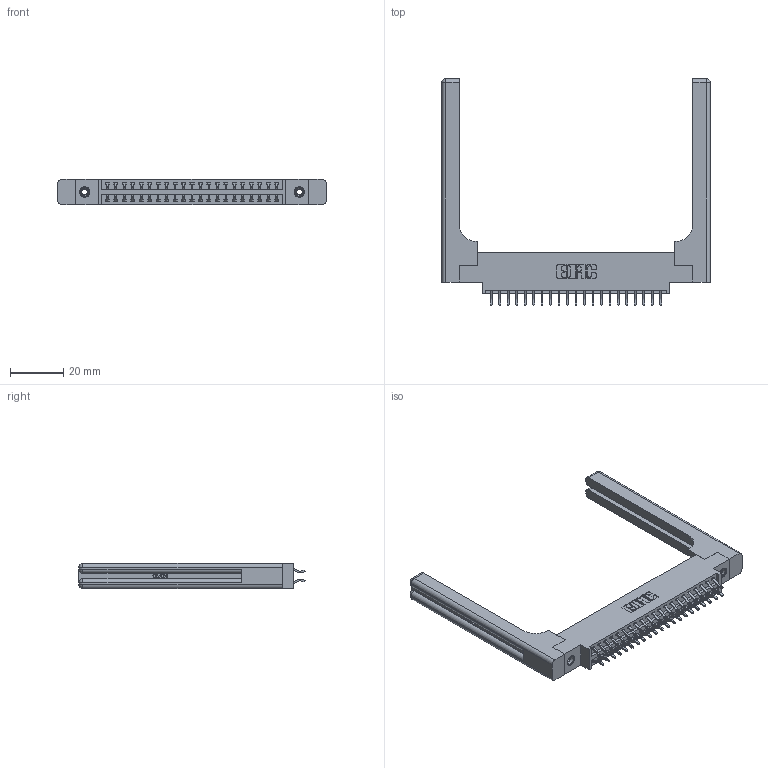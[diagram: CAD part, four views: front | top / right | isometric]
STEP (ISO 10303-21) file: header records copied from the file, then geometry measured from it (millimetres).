
FILE_DESCRIPTION (( 'STEP AP203' ), '1' );
FILE_NAME ('346-042-556-858.STEP', '2022-05-20T05:15:51', ( '' ), ( '' ), 'SwSTEP 2.0', 'SolidWorks 2020', '' );
FILE_SCHEMA (( 'CONFIG_CONTROL_DESIGN' ));
Length unit declared in the file: inch
Products named in the file (5): 346-220-058_345-220-058; 345-292-001_556 Tail; 345-250-001_345-250-001-102; 346-042-556-858; 346 Part_0.170 Offset - 0.156 Dia-TH
Assembly tree (47 placements, depth 2):
  346-042-556-858
    346 Part_0.170 Offset - 0.156 Dia-TH
    345-292-001_556 Tail  x42
    345-250-001_345-250-001-102  x2
    346-220-058_345-220-058  x2
Bounding box: 100.74 x 84.84 x 9.4 mm (x, y, z)
Volume: 16979.8 mm3; surface area: 17856.4 mm2
Topology: 47 solids, 47 shells, 2832 faces, 8309 edges, 5462 vertices
Faces by surface type: plane 1880, cylinder 892, bspline 36, cone 12, sphere 8, torus 4
Entity records: 22482 total; most frequent: CARTESIAN_POINT 4763, ORIENTED_EDGE 3480, DIRECTION 3168, EDGE_CURVE 1740, LINE 1424, VECTOR 1424, VERTEX_POINT 1150, AXIS2_PLACEMENT_3D 872
